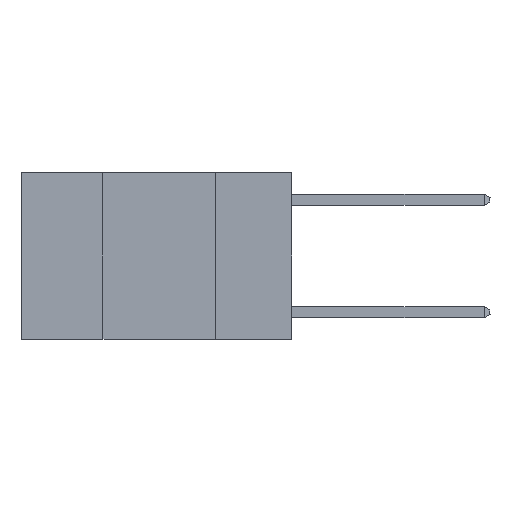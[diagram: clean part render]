
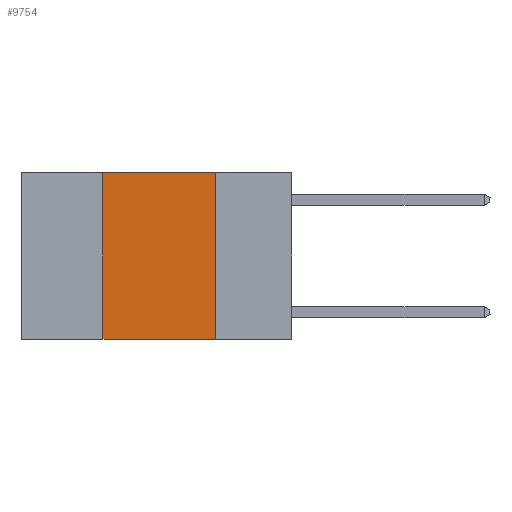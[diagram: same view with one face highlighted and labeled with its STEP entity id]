
A CAD part, left-side view. The second image highlights one B-rep face of the part: STEP entity #9754.
In plain terms, the highlighted planar face has unit normal (-1, 0, 0).
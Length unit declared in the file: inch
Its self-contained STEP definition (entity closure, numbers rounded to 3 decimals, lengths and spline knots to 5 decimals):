
#995 = CARTESIAN_POINT ( 'NONE',  ( 0., 0.6, 0. ) ) ;
#2086 = AXIS2_PLACEMENT_3D ( 'NONE', #8196, #19975, #4881 ) ;
#2627 = DIRECTION ( 'NONE',  ( 0., -1., 0. ) ) ;
#2977 = LINE ( 'NONE', #4853, #8079 ) ;
#3500 = EDGE_CURVE ( 'NONE', #11651, #16424, #17739, .T. ) ;
#4752 = VECTOR ( 'NONE', #10552, 39.37008 ) ;
#4853 = CARTESIAN_POINT ( 'NONE',  ( 0., 0.17, 0. ) ) ;
#4881 = DIRECTION ( 'NONE',  ( 0., 0., -1. ) ) ;
#5371 = ORIENTED_EDGE ( 'NONE', *, *, #20074, .F. ) ;
#7272 = EDGE_CURVE ( 'NONE', #16424, #18963, #2977, .T. ) ;
#8079 = VECTOR ( 'NONE', #13356, 39.37008 ) ;
#8196 = CARTESIAN_POINT ( 'NONE',  ( 0., 0.6, 0. ) ) ;
#8418 = CARTESIAN_POINT ( 'NONE',  ( 0., 0.42, -0.37 ) ) ;
#8646 = CARTESIAN_POINT ( 'NONE',  ( 0., 0.42, 0. ) ) ;
#9565 = ORIENTED_EDGE ( 'NONE', *, *, #7272, .F. ) ;
#9664 = FACE_OUTER_BOUND ( 'NONE', #19799, .T. ) ;
#9754 = ADVANCED_FACE ( 'NONE', ( #9664 ), #14719, .F. ) ;
#10552 = DIRECTION ( 'NONE',  ( 0., 0., 1. ) ) ;
#10788 = CARTESIAN_POINT ( 'NONE',  ( 0., 0.17, 0. ) ) ;
#10800 = ORIENTED_EDGE ( 'NONE', *, *, #20479, .T. ) ;
#11651 = VERTEX_POINT ( 'NONE', #11894 ) ;
#11758 = LINE ( 'NONE', #8646, #4752 ) ;
#11894 = CARTESIAN_POINT ( 'NONE',  ( 0., 0.42, 0. ) ) ;
#12066 = LINE ( 'NONE', #15438, #12516 ) ;
#12516 = VECTOR ( 'NONE', #18872, 39.37008 ) ;
#12912 = CARTESIAN_POINT ( 'NONE',  ( 0., 0.17, -0.37 ) ) ;
#13356 = DIRECTION ( 'NONE',  ( 0., 0., -1. ) ) ;
#13537 = VERTEX_POINT ( 'NONE', #8418 ) ;
#14719 = PLANE ( 'NONE',  #2086 ) ;
#15438 = CARTESIAN_POINT ( 'NONE',  ( 0., 0.6, -0.37 ) ) ;
#16424 = VERTEX_POINT ( 'NONE', #10788 ) ;
#17739 = LINE ( 'NONE', #995, #18075 ) ;
#18075 = VECTOR ( 'NONE', #2627, 39.37008 ) ;
#18872 = DIRECTION ( 'NONE',  ( 0., -1., 0. ) ) ;
#18963 = VERTEX_POINT ( 'NONE', #12912 ) ;
#19799 = EDGE_LOOP ( 'NONE', ( #9565, #20777, #5371, #10800 ) ) ;
#19975 = DIRECTION ( 'NONE',  ( 1., 0., 0. ) ) ;
#20074 = EDGE_CURVE ( 'NONE', #13537, #11651, #11758, .T. ) ;
#20479 = EDGE_CURVE ( 'NONE', #13537, #18963, #12066, .T. ) ;
#20777 = ORIENTED_EDGE ( 'NONE', *, *, #3500, .F. ) ;
